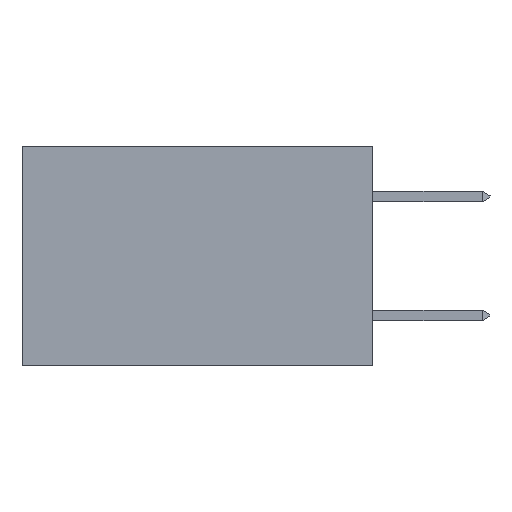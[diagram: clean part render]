
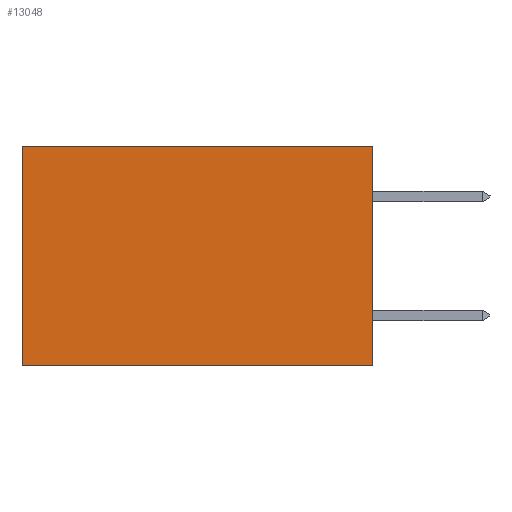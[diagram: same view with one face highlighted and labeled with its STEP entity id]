
A CAD part, left-side view. The second image highlights one B-rep face of the part: STEP entity #13048.
In plain terms, the highlighted planar face has unit normal (-1, 0, 0).
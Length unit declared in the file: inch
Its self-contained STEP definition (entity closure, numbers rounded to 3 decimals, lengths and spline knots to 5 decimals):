
#525 = DIRECTION ( 'NONE',  ( 0., 0., -1. ) ) ;
#1437 = VECTOR ( 'NONE', #13720, 39.37008 ) ;
#1493 = CARTESIAN_POINT ( 'NONE',  ( 0.277, 0.59, -0.37 ) ) ;
#2396 = VECTOR ( 'NONE', #525, 39.37008 ) ;
#2524 = ORIENTED_EDGE ( 'NONE', *, *, #6093, .F. ) ;
#2883 = DIRECTION ( 'NONE',  ( 1., 0., 0. ) ) ;
#3459 = VERTEX_POINT ( 'NONE', #10211 ) ;
#3580 = EDGE_CURVE ( 'NONE', #3459, #9232, #16975, .T. ) ;
#5790 = DIRECTION ( 'NONE',  ( 0., 1., 0. ) ) ;
#5972 = LINE ( 'NONE', #15958, #13308 ) ;
#6093 = EDGE_CURVE ( 'NONE', #9725, #9232, #9488, .T. ) ;
#6553 = ORIENTED_EDGE ( 'NONE', *, *, #8747, .F. ) ;
#7159 = AXIS2_PLACEMENT_3D ( 'NONE', #11798, #2883, #13227 ) ;
#7230 = VERTEX_POINT ( 'NONE', #15035 ) ;
#7461 = DIRECTION ( 'NONE',  ( 0., 0., -1. ) ) ;
#7500 = CARTESIAN_POINT ( 'NONE',  ( 0.277, 0.59, -0.37 ) ) ;
#8747 = EDGE_CURVE ( 'NONE', #7230, #9725, #18006, .T. ) ;
#9232 = VERTEX_POINT ( 'NONE', #1493 ) ;
#9488 = LINE ( 'NONE', #14608, #1437 ) ;
#9725 = VERTEX_POINT ( 'NONE', #9913 ) ;
#9913 = CARTESIAN_POINT ( 'NONE',  ( 0.277, 0., -0.37 ) ) ;
#10211 = CARTESIAN_POINT ( 'NONE',  ( 0.277, 0.59, 0. ) ) ;
#11029 = CARTESIAN_POINT ( 'NONE',  ( 0.277, 0., -0.37 ) ) ;
#11798 = CARTESIAN_POINT ( 'NONE',  ( 0.277, 0., -0.37 ) ) ;
#13048 = ADVANCED_FACE ( 'NONE', ( #15696 ), #18927, .F. ) ;
#13164 = VECTOR ( 'NONE', #7461, 39.37008 ) ;
#13227 = DIRECTION ( 'NONE',  ( 0., 0., -1. ) ) ;
#13308 = VECTOR ( 'NONE', #5790, 39.37008 ) ;
#13720 = DIRECTION ( 'NONE',  ( 0., 1., 0. ) ) ;
#13875 = ORIENTED_EDGE ( 'NONE', *, *, #3580, .T. ) ;
#14298 = ORIENTED_EDGE ( 'NONE', *, *, #17185, .T. ) ;
#14608 = CARTESIAN_POINT ( 'NONE',  ( 0.277, 0., -0.37 ) ) ;
#15035 = CARTESIAN_POINT ( 'NONE',  ( 0.277, 0., 0. ) ) ;
#15696 = FACE_OUTER_BOUND ( 'NONE', #17037, .T. ) ;
#15958 = CARTESIAN_POINT ( 'NONE',  ( 0.277, 0., 0. ) ) ;
#16975 = LINE ( 'NONE', #7500, #13164 ) ;
#17037 = EDGE_LOOP ( 'NONE', ( #13875, #2524, #6553, #14298 ) ) ;
#17185 = EDGE_CURVE ( 'NONE', #7230, #3459, #5972, .T. ) ;
#18006 = LINE ( 'NONE', #11029, #2396 ) ;
#18927 = PLANE ( 'NONE',  #7159 ) ;
